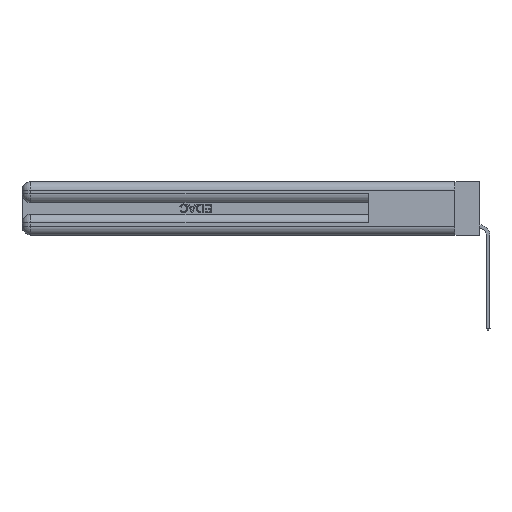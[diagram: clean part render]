
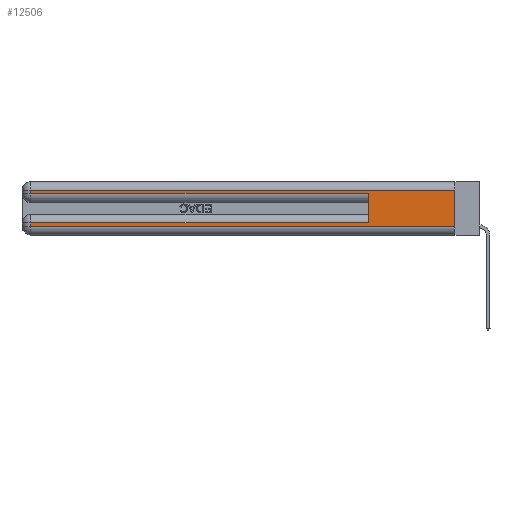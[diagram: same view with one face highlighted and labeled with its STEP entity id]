
A CAD part, left-side view. The second image highlights one B-rep face of the part: STEP entity #12506.
In plain terms, the highlighted planar face has unit normal (-1, 0, 0).
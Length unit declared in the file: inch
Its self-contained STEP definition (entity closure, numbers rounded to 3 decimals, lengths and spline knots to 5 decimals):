
#223 = LINE ( 'NONE', #19619, #14419 ) ;
#966 = LINE ( 'NONE', #10672, #26767 ) ;
#1220 = EDGE_LOOP ( 'NONE', ( #30447, #20813, #5122, #16909, #21329, #31390, #11495, #26163 ) ) ;
#2342 = CARTESIAN_POINT ( 'NONE',  ( 0., 0.6, 0.085 ) ) ;
#2496 = EDGE_CURVE ( 'NONE', #21736, #12131, #10401, .T. ) ;
#2519 = DIRECTION ( 'NONE',  ( 0., -1., 0. ) ) ;
#2857 = CARTESIAN_POINT ( 'NONE',  ( 0., 0.6, 0.285 ) ) ;
#3166 = EDGE_CURVE ( 'NONE', #26739, #16994, #223, .T. ) ;
#4005 = VERTEX_POINT ( 'NONE', #9298 ) ;
#4789 = EDGE_CURVE ( 'NONE', #12131, #4005, #966, .T. ) ;
#4900 = CARTESIAN_POINT ( 'NONE',  ( 0., 0., 0.285 ) ) ;
#5122 = ORIENTED_EDGE ( 'NONE', *, *, #4789, .T. ) ;
#5718 = VECTOR ( 'NONE', #12480, 39.37008 ) ;
#7275 = LINE ( 'NONE', #4900, #26237 ) ;
#7521 = DIRECTION ( 'NONE',  ( 0., 0., 1. ) ) ;
#8644 = VECTOR ( 'NONE', #19695, 39.37008 ) ;
#9298 = CARTESIAN_POINT ( 'NONE',  ( 0., 2.94, 0.285 ) ) ;
#9535 = EDGE_CURVE ( 'NONE', #26739, #19073, #17236, .T. ) ;
#9587 = CARTESIAN_POINT ( 'NONE',  ( 0., 2.94, 0.37 ) ) ;
#9924 = CARTESIAN_POINT ( 'NONE',  ( 0., 0., 0.31 ) ) ;
#10401 = LINE ( 'NONE', #9924, #17416 ) ;
#10672 = CARTESIAN_POINT ( 'NONE',  ( 0., 2.94, 0.37 ) ) ;
#11495 = ORIENTED_EDGE ( 'NONE', *, *, #23113, .T. ) ;
#11829 = EDGE_CURVE ( 'NONE', #21736, #24963, #22067, .T. ) ;
#12131 = VERTEX_POINT ( 'NONE', #24062 ) ;
#12480 = DIRECTION ( 'NONE',  ( 0., 1., 0. ) ) ;
#12482 = DIRECTION ( 'NONE',  ( 0., 1., 0. ) ) ;
#12506 = ADVANCED_FACE ( 'NONE', ( #26245 ), #31321, .F. ) ;
#12755 = DIRECTION ( 'NONE',  ( 0., 0., -1. ) ) ;
#13148 = EDGE_CURVE ( 'NONE', #4005, #16994, #7275, .T. ) ;
#14419 = VECTOR ( 'NONE', #7521, 39.37008 ) ;
#14843 = LINE ( 'NONE', #9587, #18962 ) ;
#14917 = DIRECTION ( 'NONE',  ( 0., 0., -1. ) ) ;
#15252 = LINE ( 'NONE', #29385, #8644 ) ;
#16236 = DIRECTION ( 'NONE',  ( 0., 0., -1. ) ) ;
#16653 = CARTESIAN_POINT ( 'NONE',  ( 0., 2.94, 0.06 ) ) ;
#16909 = ORIENTED_EDGE ( 'NONE', *, *, #13148, .T. ) ;
#16994 = VERTEX_POINT ( 'NONE', #2857 ) ;
#17236 = LINE ( 'NONE', #29309, #5718 ) ;
#17363 = VERTEX_POINT ( 'NONE', #16653 ) ;
#17416 = VECTOR ( 'NONE', #12482, 39.37008 ) ;
#18962 = VECTOR ( 'NONE', #29140, 39.37008 ) ;
#19073 = VERTEX_POINT ( 'NONE', #25608 ) ;
#19619 = CARTESIAN_POINT ( 'NONE',  ( 0., 0.6, 0.145 ) ) ;
#19695 = DIRECTION ( 'NONE',  ( 0., -1., 0. ) ) ;
#20813 = ORIENTED_EDGE ( 'NONE', *, *, #2496, .T. ) ;
#21320 = DIRECTION ( 'NONE',  ( 1., 0., 0. ) ) ;
#21329 = ORIENTED_EDGE ( 'NONE', *, *, #3166, .F. ) ;
#21643 = CARTESIAN_POINT ( 'NONE',  ( 0., 0., 0.37 ) ) ;
#21736 = VERTEX_POINT ( 'NONE', #22882 ) ;
#22067 = LINE ( 'NONE', #26522, #29213 ) ;
#22882 = CARTESIAN_POINT ( 'NONE',  ( 0., 0., 0.31 ) ) ;
#23113 = EDGE_CURVE ( 'NONE', #19073, #17363, #14843, .T. ) ;
#24062 = CARTESIAN_POINT ( 'NONE',  ( 0., 2.94, 0.31 ) ) ;
#24963 = VERTEX_POINT ( 'NONE', #29725 ) ;
#25608 = CARTESIAN_POINT ( 'NONE',  ( 0., 2.94, 0.085 ) ) ;
#26163 = ORIENTED_EDGE ( 'NONE', *, *, #26513, .T. ) ;
#26237 = VECTOR ( 'NONE', #2519, 39.37008 ) ;
#26245 = FACE_OUTER_BOUND ( 'NONE', #1220, .T. ) ;
#26513 = EDGE_CURVE ( 'NONE', #17363, #24963, #15252, .T. ) ;
#26522 = CARTESIAN_POINT ( 'NONE',  ( 0., 0., 0.37 ) ) ;
#26739 = VERTEX_POINT ( 'NONE', #2342 ) ;
#26767 = VECTOR ( 'NONE', #12755, 39.37008 ) ;
#29140 = DIRECTION ( 'NONE',  ( 0., 0., -1. ) ) ;
#29213 = VECTOR ( 'NONE', #14917, 39.37008 ) ;
#29309 = CARTESIAN_POINT ( 'NONE',  ( 0., 0., 0.085 ) ) ;
#29385 = CARTESIAN_POINT ( 'NONE',  ( 0., 0., 0.06 ) ) ;
#29725 = CARTESIAN_POINT ( 'NONE',  ( 0., 0., 0.06 ) ) ;
#29752 = AXIS2_PLACEMENT_3D ( 'NONE', #21643, #21320, #16236 ) ;
#30447 = ORIENTED_EDGE ( 'NONE', *, *, #11829, .F. ) ;
#31321 = PLANE ( 'NONE',  #29752 ) ;
#31390 = ORIENTED_EDGE ( 'NONE', *, *, #9535, .T. ) ;
